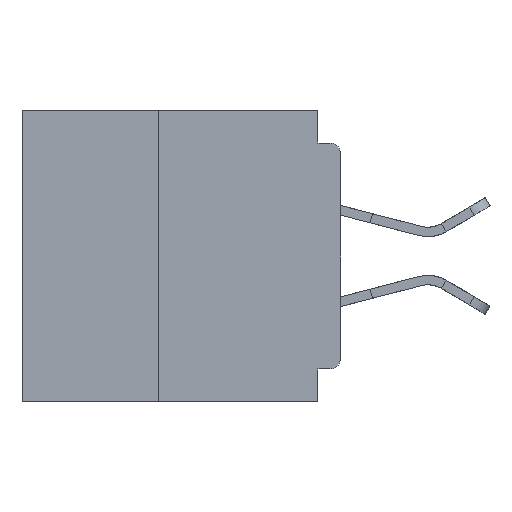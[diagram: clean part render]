
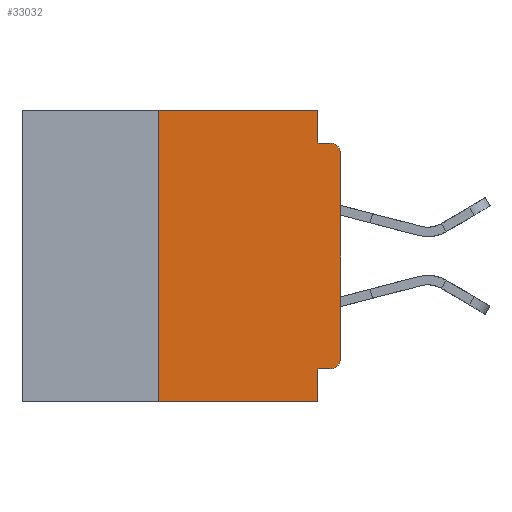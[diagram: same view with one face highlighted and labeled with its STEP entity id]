
A CAD part, left-side view. The second image highlights one B-rep face of the part: STEP entity #33032.
In plain terms, the highlighted planar face has unit normal (-1, 0, 0).
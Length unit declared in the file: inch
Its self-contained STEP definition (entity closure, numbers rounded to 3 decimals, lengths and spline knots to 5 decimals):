
#3168 = ORIENTED_EDGE ( 'NONE', *, *, #45804, .F. ) ;
#3681 = ORIENTED_EDGE ( 'NONE', *, *, #23406, .T. ) ;
#3769 = ORIENTED_EDGE ( 'NONE', *, *, #6869, .F. ) ;
#3838 = LINE ( 'NONE', #34471, #31546 ) ;
#6821 = VERTEX_POINT ( 'NONE', #14037 ) ;
#6869 = EDGE_CURVE ( 'NONE', #40327, #31325, #36036, .T. ) ;
#6928 = EDGE_CURVE ( 'NONE', #28962, #37927, #14764, .T. ) ;
#7831 = ORIENTED_EDGE ( 'NONE', *, *, #6928, .F. ) ;
#9015 = DIRECTION ( 'NONE',  ( 0., 0., -1. ) ) ;
#9310 = DIRECTION ( 'NONE',  ( 0., 0., -1. ) ) ;
#9508 = CARTESIAN_POINT ( 'NONE',  ( 0., 0.031, -0.355 ) ) ;
#9561 = ORIENTED_EDGE ( 'NONE', *, *, #29170, .T. ) ;
#10382 = EDGE_LOOP ( 'NONE', ( #3681, #41587, #14658, #3168, #22519, #3769, #18080, #14146, #7831, #9561 ) ) ;
#11359 = EDGE_CURVE ( 'NONE', #37927, #19552, #22707, .T. ) ;
#11708 = CIRCLE ( 'NONE', #45483, 0.015 ) ;
#12058 = FACE_OUTER_BOUND ( 'NONE', #10382, .T. ) ;
#13131 = EDGE_CURVE ( 'NONE', #40327, #19552, #23860, .T. ) ;
#14037 = CARTESIAN_POINT ( 'NONE',  ( 0., 0.015, -0.045 ) ) ;
#14146 = ORIENTED_EDGE ( 'NONE', *, *, #11359, .F. ) ;
#14354 = VECTOR ( 'NONE', #20030, 39.37008 ) ;
#14658 = ORIENTED_EDGE ( 'NONE', *, *, #42229, .F. ) ;
#14764 = LINE ( 'NONE', #35950, #32623 ) ;
#14830 = DIRECTION ( 'NONE',  ( 1., 0., 0. ) ) ;
#14965 = VERTEX_POINT ( 'NONE', #45367 ) ;
#17205 = CARTESIAN_POINT ( 'NONE',  ( 0., 0., -0.06 ) ) ;
#18080 = ORIENTED_EDGE ( 'NONE', *, *, #13131, .T. ) ;
#18269 = PLANE ( 'NONE',  #23523 ) ;
#18350 = AXIS2_PLACEMENT_3D ( 'NONE', #40200, #18689, #43854 ) ;
#18689 = DIRECTION ( 'NONE',  ( -1., 0., 0. ) ) ;
#19552 = VERTEX_POINT ( 'NONE', #33583 ) ;
#20030 = DIRECTION ( 'NONE',  ( 0., -1., 0. ) ) ;
#20693 = DIRECTION ( 'NONE',  ( -1., 0., 0. ) ) ;
#21564 = DIRECTION ( 'NONE',  ( 0., 0., 1. ) ) ;
#21596 = LINE ( 'NONE', #30731, #40700 ) ;
#22519 = ORIENTED_EDGE ( 'NONE', *, *, #37182, .F. ) ;
#22707 = LINE ( 'NONE', #37825, #40697 ) ;
#22902 = VECTOR ( 'NONE', #44258, 39.37008 ) ;
#23406 = EDGE_CURVE ( 'NONE', #26491, #45324, #21596, .T. ) ;
#23523 = AXIS2_PLACEMENT_3D ( 'NONE', #36254, #14830, #39937 ) ;
#23824 = CARTESIAN_POINT ( 'NONE',  ( 0., 0.25, -0.4 ) ) ;
#23860 = LINE ( 'NONE', #45203, #14354 ) ;
#26491 = VERTEX_POINT ( 'NONE', #40851 ) ;
#28962 = VERTEX_POINT ( 'NONE', #31024 ) ;
#29108 = CARTESIAN_POINT ( 'NONE',  ( 0., 0.031, 0. ) ) ;
#29170 = EDGE_CURVE ( 'NONE', #28962, #26491, #33614, .T. ) ;
#30027 = EDGE_CURVE ( 'NONE', #45324, #6821, #11708, .T. ) ;
#30731 = CARTESIAN_POINT ( 'NONE',  ( 0., 0., 0. ) ) ;
#31024 = CARTESIAN_POINT ( 'NONE',  ( 0., 0.015, -0.355 ) ) ;
#31325 = VERTEX_POINT ( 'NONE', #46579 ) ;
#31546 = VECTOR ( 'NONE', #9310, 39.37008 ) ;
#31963 = LINE ( 'NONE', #34031, #42743 ) ;
#32623 = VECTOR ( 'NONE', #43429, 39.37008 ) ;
#33032 = ADVANCED_FACE ( 'NONE', ( #12058 ), #18269, .F. ) ;
#33583 = CARTESIAN_POINT ( 'NONE',  ( 0., 0.031, -0.4 ) ) ;
#33614 = CIRCLE ( 'NONE', #18350, 0.015 ) ;
#34031 = CARTESIAN_POINT ( 'NONE',  ( 0., 0., -0.045 ) ) ;
#34327 = DIRECTION ( 'NONE',  ( 0., 0., 1. ) ) ;
#34471 = CARTESIAN_POINT ( 'NONE',  ( 0., 0.031, 0. ) ) ;
#35950 = CARTESIAN_POINT ( 'NONE',  ( 0., 0., -0.355 ) ) ;
#36036 = LINE ( 'NONE', #46776, #44577 ) ;
#36254 = CARTESIAN_POINT ( 'NONE',  ( 0., 0.437, 0. ) ) ;
#36775 = CARTESIAN_POINT ( 'NONE',  ( 0., 0.437, 0. ) ) ;
#37182 = EDGE_CURVE ( 'NONE', #31325, #44372, #39771, .T. ) ;
#37679 = DIRECTION ( 'NONE',  ( 0., -1., 0. ) ) ;
#37825 = CARTESIAN_POINT ( 'NONE',  ( 0., 0.031, -0.4 ) ) ;
#37927 = VERTEX_POINT ( 'NONE', #9508 ) ;
#39771 = LINE ( 'NONE', #36775, #22902 ) ;
#39937 = DIRECTION ( 'NONE',  ( 0., 0., -1. ) ) ;
#40200 = CARTESIAN_POINT ( 'NONE',  ( 0., 0.015, -0.34 ) ) ;
#40327 = VERTEX_POINT ( 'NONE', #23824 ) ;
#40697 = VECTOR ( 'NONE', #9015, 39.37008 ) ;
#40700 = VECTOR ( 'NONE', #34327, 39.37008 ) ;
#40851 = CARTESIAN_POINT ( 'NONE',  ( 0., 0., -0.34 ) ) ;
#41587 = ORIENTED_EDGE ( 'NONE', *, *, #30027, .T. ) ;
#42217 = CARTESIAN_POINT ( 'NONE',  ( 0., 0.015, -0.06 ) ) ;
#42229 = EDGE_CURVE ( 'NONE', #14965, #6821, #31963, .T. ) ;
#42743 = VECTOR ( 'NONE', #37679, 39.37008 ) ;
#43429 = DIRECTION ( 'NONE',  ( 0., 1., 0. ) ) ;
#43854 = DIRECTION ( 'NONE',  ( 0., 0., -1. ) ) ;
#44258 = DIRECTION ( 'NONE',  ( 0., -1., 0. ) ) ;
#44372 = VERTEX_POINT ( 'NONE', #29108 ) ;
#44577 = VECTOR ( 'NONE', #21564, 39.37008 ) ;
#45203 = CARTESIAN_POINT ( 'NONE',  ( 0., 0.437, -0.4 ) ) ;
#45324 = VERTEX_POINT ( 'NONE', #17205 ) ;
#45367 = CARTESIAN_POINT ( 'NONE',  ( 0., 0.031, -0.045 ) ) ;
#45483 = AXIS2_PLACEMENT_3D ( 'NONE', #42217, #20693, #45865 ) ;
#45804 = EDGE_CURVE ( 'NONE', #44372, #14965, #3838, .T. ) ;
#45865 = DIRECTION ( 'NONE',  ( 0., 0., -1. ) ) ;
#46579 = CARTESIAN_POINT ( 'NONE',  ( 0., 0.25, 0. ) ) ;
#46776 = CARTESIAN_POINT ( 'NONE',  ( 0., 0.25, -0.4 ) ) ;
